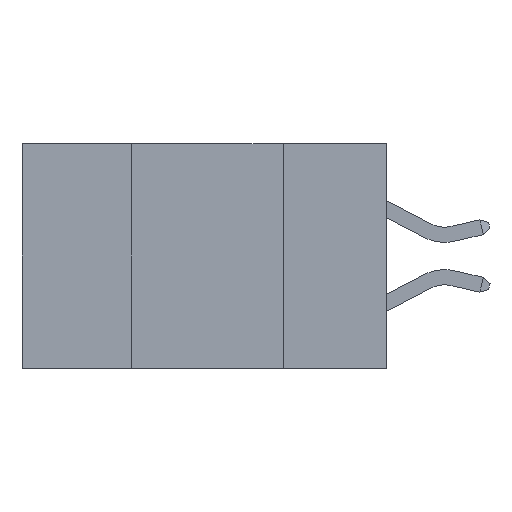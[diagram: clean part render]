
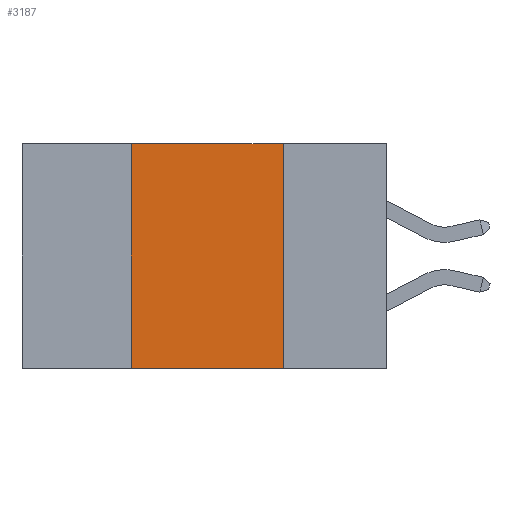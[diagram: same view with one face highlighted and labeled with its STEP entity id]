
A CAD part, left-side view. The second image highlights one B-rep face of the part: STEP entity #3187.
In plain terms, the highlighted planar face has unit normal (-1, 0, 0).
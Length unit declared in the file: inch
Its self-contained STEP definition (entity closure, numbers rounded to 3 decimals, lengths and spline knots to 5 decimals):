
#346 = VERTEX_POINT ( 'NONE', #8994 ) ;
#413 = DIRECTION ( 'NONE',  ( 1., 0., 0. ) ) ;
#744 = VERTEX_POINT ( 'NONE', #3585 ) ;
#806 = DIRECTION ( 'NONE',  ( 0., -1., 0. ) ) ;
#1292 = VERTEX_POINT ( 'NONE', #3182 ) ;
#1486 = VECTOR ( 'NONE', #7513, 39.37008 ) ;
#1819 = CARTESIAN_POINT ( 'NONE',  ( 0., 0.42, 0. ) ) ;
#2557 = LINE ( 'NONE', #4952, #1486 ) ;
#2568 = DIRECTION ( 'NONE',  ( 0., 0., 1. ) ) ;
#2585 = LINE ( 'NONE', #6022, #8313 ) ;
#2779 = LINE ( 'NONE', #1819, #7031 ) ;
#2806 = FACE_OUTER_BOUND ( 'NONE', #5342, .T. ) ;
#3105 = EDGE_CURVE ( 'NONE', #346, #744, #4785, .T. ) ;
#3182 = CARTESIAN_POINT ( 'NONE',  ( 0., 0.42, -0.37 ) ) ;
#3187 = ADVANCED_FACE ( 'NONE', ( #2806 ), #3758, .F. ) ;
#3585 = CARTESIAN_POINT ( 'NONE',  ( 0., 0.17, -0.37 ) ) ;
#3758 = PLANE ( 'NONE',  #8368 ) ;
#3816 = ORIENTED_EDGE ( 'NONE', *, *, #8465, .F. ) ;
#4785 = LINE ( 'NONE', #10561, #5592 ) ;
#4952 = CARTESIAN_POINT ( 'NONE',  ( 0., 0.6, -0.37 ) ) ;
#5342 = EDGE_LOOP ( 'NONE', ( #10729, #3816, #7941, #5666 ) ) ;
#5545 = CARTESIAN_POINT ( 'NONE',  ( 0., 0.6, 0. ) ) ;
#5592 = VECTOR ( 'NONE', #9791, 39.37008 ) ;
#5666 = ORIENTED_EDGE ( 'NONE', *, *, #9488, .T. ) ;
#6022 = CARTESIAN_POINT ( 'NONE',  ( 0., 0.6, 0. ) ) ;
#6265 = EDGE_CURVE ( 'NONE', #1292, #8091, #2779, .T. ) ;
#7031 = VECTOR ( 'NONE', #2568, 39.37008 ) ;
#7513 = DIRECTION ( 'NONE',  ( 0., -1., 0. ) ) ;
#7941 = ORIENTED_EDGE ( 'NONE', *, *, #6265, .F. ) ;
#8091 = VERTEX_POINT ( 'NONE', #9084 ) ;
#8313 = VECTOR ( 'NONE', #806, 39.37008 ) ;
#8368 = AXIS2_PLACEMENT_3D ( 'NONE', #5545, #413, #9147 ) ;
#8465 = EDGE_CURVE ( 'NONE', #8091, #346, #2585, .T. ) ;
#8994 = CARTESIAN_POINT ( 'NONE',  ( 0., 0.17, 0. ) ) ;
#9084 = CARTESIAN_POINT ( 'NONE',  ( 0., 0.42, 0. ) ) ;
#9147 = DIRECTION ( 'NONE',  ( 0., 0., -1. ) ) ;
#9488 = EDGE_CURVE ( 'NONE', #1292, #744, #2557, .T. ) ;
#9791 = DIRECTION ( 'NONE',  ( 0., 0., -1. ) ) ;
#10561 = CARTESIAN_POINT ( 'NONE',  ( 0., 0.17, 0. ) ) ;
#10729 = ORIENTED_EDGE ( 'NONE', *, *, #3105, .F. ) ;
